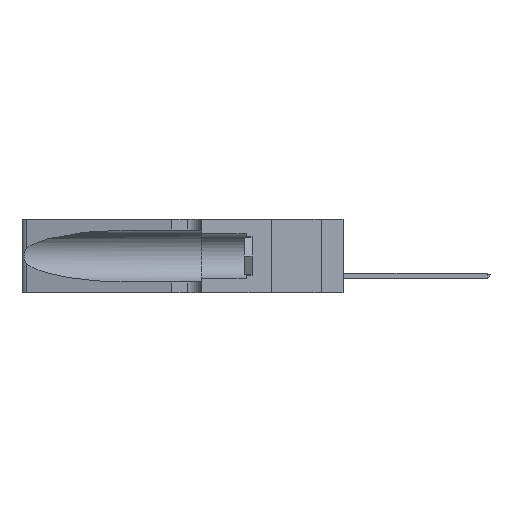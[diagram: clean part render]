
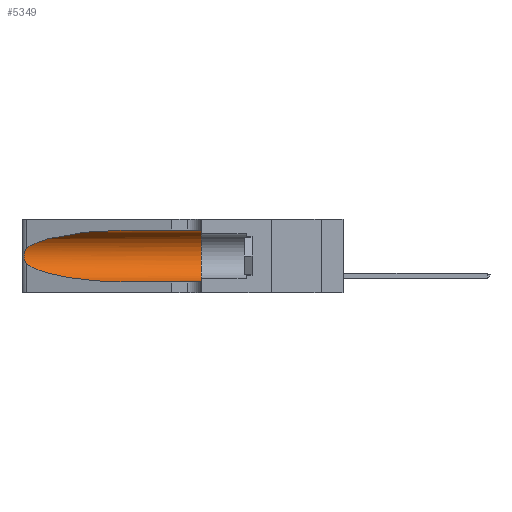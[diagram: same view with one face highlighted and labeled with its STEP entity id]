
A CAD part, left-side view. The second image highlights one B-rep face of the part: STEP entity #5349.
In plain terms, the highlighted cylindrical face has radius 3.308 mm (diameter 6.617 mm), a partial arc.
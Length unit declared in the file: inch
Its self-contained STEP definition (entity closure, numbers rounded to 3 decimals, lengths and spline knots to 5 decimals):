
#40 = VERTEX_POINT ( 'NONE', #19660 ) ;
#189 = CARTESIAN_POINT ( 'NONE',  ( 0.1305, 1.61858, 0.31525 ) ) ;
#873 = EDGE_LOOP ( 'NONE', ( #5573, #5069, #8004, #15902, #19690, #15240 ) ) ;
#1101 = CARTESIAN_POINT ( 'NONE',  ( 0.26075, 1.23896, 0.178 ) ) ;
#1127 = CARTESIAN_POINT ( 'NONE',  ( 0.1305, 0.72297, 0.05475 ) ) ;
#1181 = CARTESIAN_POINT ( 'NONE',  ( 0.25487, 1.22718, 0.22369 ) ) ;
#1353 = DIRECTION ( 'NONE',  ( 0., -1., 0. ) ) ;
#1650 = EDGE_CURVE ( 'NONE', #40, #25324, #3462, .T. ) ;
#2681 = CARTESIAN_POINT ( 'NONE',  ( 0.25487, 1.22718, 0.22369 ) ) ;
#2915 = CARTESIAN_POINT ( 'NONE',  ( 0.1305, 1.61858, 0.185 ) ) ;
#3462 =( BOUNDED_CURVE ( )  B_SPLINE_CURVE ( 3, ( #21334, #16801, #23674, #1181 ),
 .UNSPECIFIED., .F., .F. ) 
 B_SPLINE_CURVE_WITH_KNOTS ( ( 4, 4 ),
 ( 1.5708, 2.84003 ),
 .UNSPECIFIED. ) 
 CURVE ( )  GEOMETRIC_REPRESENTATION_ITEM ( )  RATIONAL_B_SPLINE_CURVE ( ( 1., 0.87, 0.87, 1. ) ) 
 REPRESENTATION_ITEM ( '' )  );
#5038 = CARTESIAN_POINT ( 'NONE',  ( 0.25487, 1.22718, 0.14631 ) ) ;
#5069 = ORIENTED_EDGE ( 'NONE', *, *, #21184, .T. ) ;
#5349 = ADVANCED_FACE ( 'NONE', ( #20612 ), #12625, .F. ) ;
#5526 = AXIS2_PLACEMENT_3D ( 'NONE', #22434, #13609, #6988 ) ;
#5573 = ORIENTED_EDGE ( 'NONE', *, *, #1650, .T. ) ;
#5943 = CARTESIAN_POINT ( 'NONE',  ( 0.25487, 1.22718, 0.14631 ) ) ;
#6395 = AXIS2_PLACEMENT_3D ( 'NONE', #2915, #18251, #7331 ) ;
#6561 = EDGE_CURVE ( 'NONE', #40, #20506, #22942, .T. ) ;
#6988 = DIRECTION ( 'NONE',  ( 0., 0., 1. ) ) ;
#7331 = DIRECTION ( 'NONE',  ( 0., 0., -1. ) ) ;
#7885 = CARTESIAN_POINT ( 'NONE',  ( 0.1305, 1.61858, 0.05475 ) ) ;
#7934 = CARTESIAN_POINT ( 'NONE',  ( 0.26018, 1.23835, 0.19895 ) ) ;
#8004 = ORIENTED_EDGE ( 'NONE', *, *, #10232, .T. ) ;
#8576 = CARTESIAN_POINT ( 'NONE',  ( 0.1305, 0.35, 0.05475 ) ) ;
#9044 = VECTOR ( 'NONE', #24333, 39.37008 ) ;
#9316 = CARTESIAN_POINT ( 'NONE',  ( 0.18966, 0.96281, 0.05475 ) ) ;
#9809 = CARTESIAN_POINT ( 'NONE',  ( 0.25555, 1.22993, 0.14849 ) ) ;
#9937 = EDGE_CURVE ( 'NONE', #20506, #19029, #21700, .T. ) ;
#10232 = EDGE_CURVE ( 'NONE', #16371, #27696, #20550, .T. ) ;
#12148 = CARTESIAN_POINT ( 'NONE',  ( 0.25854, 1.2359, 0.20912 ) ) ;
#12439 = CARTESIAN_POINT ( 'NONE',  ( 0.25639, 1.23184, 0.21858 ) ) ;
#12625 = CYLINDRICAL_SURFACE ( 'NONE', #6395, 0.13025 ) ;
#13609 = DIRECTION ( 'NONE',  ( 0., 1., 0. ) ) ;
#14894 = EDGE_CURVE ( 'NONE', #27696, #19029, #27335, .T. ) ;
#15240 = ORIENTED_EDGE ( 'NONE', *, *, #6561, .F. ) ;
#15578 = CARTESIAN_POINT ( 'NONE',  ( 0.1305, 0.35, 0.31525 ) ) ;
#15902 = ORIENTED_EDGE ( 'NONE', *, *, #14894, .T. ) ;
#15938 = B_SPLINE_CURVE_WITH_KNOTS ( 'NONE', 3,
 ( #16354, #24967, #12439, #19053, #12148, #7934, #27614, #1101, #21246, #23105, #16911, #16721, #9809, #27700 ),
 .UNSPECIFIED., .F., .F.,
 ( 4, 2, 2, 2, 2, 2, 4 ),
 ( 0., 0.00027, 0.00053, 0.00107, 0.0016, 0.00187, 0.00214 ),
 .UNSPECIFIED. ) ;
#16139 = CARTESIAN_POINT ( 'NONE',  ( 0.2373, 1.15595, 0.08982 ) ) ;
#16354 = CARTESIAN_POINT ( 'NONE',  ( 0.25487, 1.22718, 0.22369 ) ) ;
#16371 = VERTEX_POINT ( 'NONE', #5943 ) ;
#16721 = CARTESIAN_POINT ( 'NONE',  ( 0.25639, 1.23186, 0.15144 ) ) ;
#16801 = CARTESIAN_POINT ( 'NONE',  ( 0.18966, 0.96281, 0.31525 ) ) ;
#16911 = CARTESIAN_POINT ( 'NONE',  ( 0.25789, 1.23486, 0.15765 ) ) ;
#18251 = DIRECTION ( 'NONE',  ( 0., -1., 0. ) ) ;
#19029 = VERTEX_POINT ( 'NONE', #8576 ) ;
#19053 = CARTESIAN_POINT ( 'NONE',  ( 0.25787, 1.23484, 0.2124 ) ) ;
#19660 = CARTESIAN_POINT ( 'NONE',  ( 0.1305, 0.72297, 0.31525 ) ) ;
#19690 = ORIENTED_EDGE ( 'NONE', *, *, #9937, .F. ) ;
#20506 = VERTEX_POINT ( 'NONE', #15578 ) ;
#20550 =( BOUNDED_CURVE ( )  B_SPLINE_CURVE ( 3, ( #5038, #16139, #9316, #24839 ),
 .UNSPECIFIED., .F., .F. ) 
 B_SPLINE_CURVE_WITH_KNOTS ( ( 4, 4 ),
 ( 3.44316, 4.71239 ),
 .UNSPECIFIED. ) 
 CURVE ( )  GEOMETRIC_REPRESENTATION_ITEM ( )  RATIONAL_B_SPLINE_CURVE ( ( 1., 0.87, 0.87, 1. ) ) 
 REPRESENTATION_ITEM ( '' )  );
#20612 = FACE_OUTER_BOUND ( 'NONE', #873, .T. ) ;
#21184 = EDGE_CURVE ( 'NONE', #25324, #16371, #15938, .T. ) ;
#21246 = CARTESIAN_POINT ( 'NONE',  ( 0.26017, 1.23833, 0.17102 ) ) ;
#21334 = CARTESIAN_POINT ( 'NONE',  ( 0.1305, 0.72297, 0.31525 ) ) ;
#21700 = CIRCLE ( 'NONE', #5526, 0.13025 ) ;
#22434 = CARTESIAN_POINT ( 'NONE',  ( 0.1305, 0.35, 0.185 ) ) ;
#22942 = LINE ( 'NONE', #189, #9044 ) ;
#23105 = CARTESIAN_POINT ( 'NONE',  ( 0.25856, 1.23593, 0.16098 ) ) ;
#23674 = CARTESIAN_POINT ( 'NONE',  ( 0.2373, 1.15595, 0.28018 ) ) ;
#24333 = DIRECTION ( 'NONE',  ( 0., -1., 0. ) ) ;
#24839 = CARTESIAN_POINT ( 'NONE',  ( 0.1305, 0.72297, 0.05475 ) ) ;
#24967 = CARTESIAN_POINT ( 'NONE',  ( 0.25555, 1.22994, 0.2215 ) ) ;
#25324 = VERTEX_POINT ( 'NONE', #2681 ) ;
#25911 = VECTOR ( 'NONE', #1353, 39.37008 ) ;
#27335 = LINE ( 'NONE', #7885, #25911 ) ;
#27614 = CARTESIAN_POINT ( 'NONE',  ( 0.26075, 1.23896, 0.19203 ) ) ;
#27696 = VERTEX_POINT ( 'NONE', #1127 ) ;
#27700 = CARTESIAN_POINT ( 'NONE',  ( 0.25487, 1.22718, 0.14631 ) ) ;
